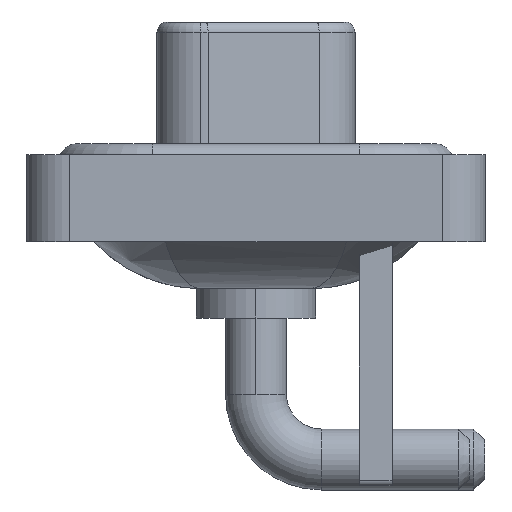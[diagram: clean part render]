
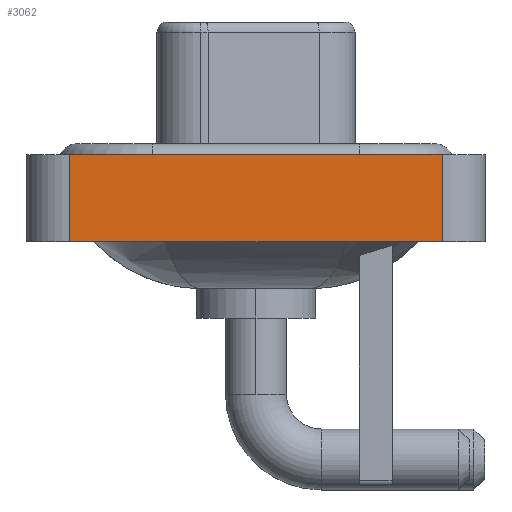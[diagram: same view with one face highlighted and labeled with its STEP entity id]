
A CAD part, left-side view. The second image highlights one B-rep face of the part: STEP entity #3062.
In plain terms, the highlighted planar face has unit normal (-1, 0, 0).
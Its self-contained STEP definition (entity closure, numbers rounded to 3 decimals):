
#335 = CARTESIAN_POINT ( 'NONE',  ( -7.3, -8.55, -3.6 ) ) ;
#1099 = DIRECTION ( 'NONE',  ( 0., -1., 0. ) ) ;
#1611 = EDGE_CURVE ( 'NONE', #6180, #11807, #4085, .T. ) ;
#2113 = CARTESIAN_POINT ( 'NONE',  ( -7.3, 8.55, 0.4 ) ) ;
#2472 = DIRECTION ( 'NONE',  ( 0., 0., 1. ) ) ;
#2608 = LINE ( 'NONE', #8753, #10934 ) ;
#2662 = CARTESIAN_POINT ( 'NONE',  ( -7.3, -8.55, 0.4 ) ) ;
#3062 = ADVANCED_FACE ( 'NONE', ( #14532 ), #8093, .T. ) ;
#3119 = LINE ( 'NONE', #4731, #15661 ) ;
#3518 = CARTESIAN_POINT ( 'NONE',  ( -7.3, 8.55, -3.6 ) ) ;
#4068 = VECTOR ( 'NONE', #2472, 1000. ) ;
#4085 = LINE ( 'NONE', #12087, #4068 ) ;
#4731 = CARTESIAN_POINT ( 'NONE',  ( -7.3, -8.55, -3.6 ) ) ;
#4790 = ORIENTED_EDGE ( 'NONE', *, *, #1611, .F. ) ;
#5175 = DIRECTION ( 'NONE',  ( 0., 0., 1. ) ) ;
#5228 = VECTOR ( 'NONE', #17669, 1000. ) ;
#6180 = VERTEX_POINT ( 'NONE', #3518 ) ;
#8093 = PLANE ( 'NONE',  #9875 ) ;
#8753 = CARTESIAN_POINT ( 'NONE',  ( -7.3, -8.55, -3.6 ) ) ;
#9645 = EDGE_CURVE ( 'NONE', #11807, #14050, #11437, .T. ) ;
#9875 = AXIS2_PLACEMENT_3D ( 'NONE', #335, #19085, #5175 ) ;
#10108 = CARTESIAN_POINT ( 'NONE',  ( -7.3, -8.55, 0.4 ) ) ;
#10468 = ORIENTED_EDGE ( 'NONE', *, *, #11668, .T. ) ;
#10650 = EDGE_LOOP ( 'NONE', ( #10468, #18397, #4790, #14045 ) ) ;
#10934 = VECTOR ( 'NONE', #1099, 1000. ) ;
#11437 = LINE ( 'NONE', #10108, #5228 ) ;
#11668 = EDGE_CURVE ( 'NONE', #16611, #14050, #3119, .T. ) ;
#11807 = VERTEX_POINT ( 'NONE', #2113 ) ;
#12087 = CARTESIAN_POINT ( 'NONE',  ( -7.3, 8.55, -3.6 ) ) ;
#12629 = DIRECTION ( 'NONE',  ( 0., 0., 1. ) ) ;
#13607 = EDGE_CURVE ( 'NONE', #6180, #16611, #2608, .T. ) ;
#14045 = ORIENTED_EDGE ( 'NONE', *, *, #13607, .T. ) ;
#14050 = VERTEX_POINT ( 'NONE', #2662 ) ;
#14532 = FACE_OUTER_BOUND ( 'NONE', #10650, .T. ) ;
#15661 = VECTOR ( 'NONE', #12629, 1000. ) ;
#16611 = VERTEX_POINT ( 'NONE', #19295 ) ;
#17669 = DIRECTION ( 'NONE',  ( 0., -1., 0. ) ) ;
#18397 = ORIENTED_EDGE ( 'NONE', *, *, #9645, .F. ) ;
#19085 = DIRECTION ( 'NONE',  ( -1., 0., 0. ) ) ;
#19295 = CARTESIAN_POINT ( 'NONE',  ( -7.3, -8.55, -3.6 ) ) ;
